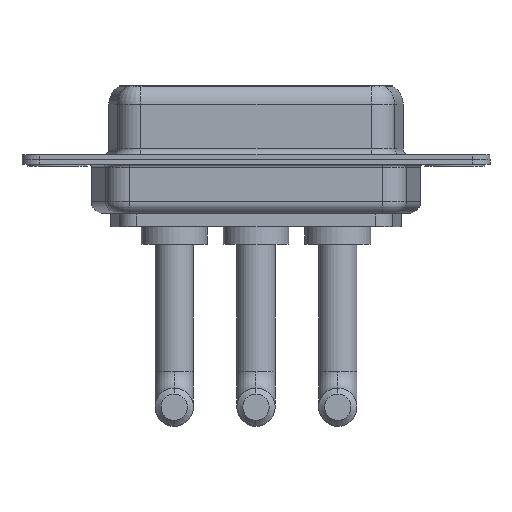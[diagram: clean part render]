
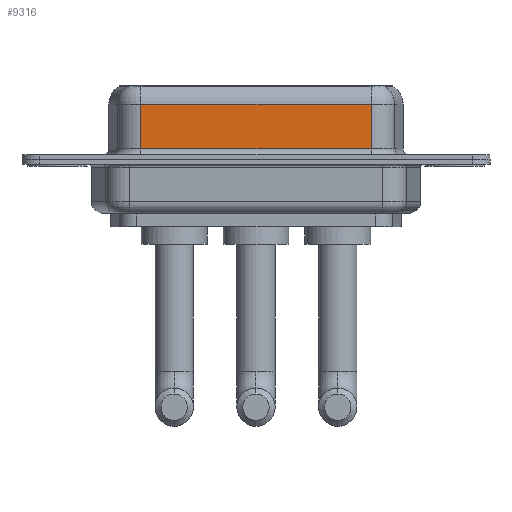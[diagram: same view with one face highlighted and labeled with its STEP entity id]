
A CAD part, front view. The second image highlights one B-rep face of the part: STEP entity #9316.
In plain terms, the highlighted planar face has unit normal (0, -1, 0).
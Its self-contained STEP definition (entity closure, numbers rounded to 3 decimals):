
#898 = PLANE ( 'NONE',  #6904 ) ;
#1173 = CARTESIAN_POINT ( 'NONE',  ( 26.287, -3.95, 0.9 ) ) ;
#2052 = ORIENTED_EDGE ( 'NONE', *, *, #4105, .T. ) ;
#2805 = CARTESIAN_POINT ( 'NONE',  ( 26.287, -3.95, 4.65 ) ) ;
#3080 = EDGE_CURVE ( 'NONE', #8100, #6720, #3349, .T. ) ;
#3349 = LINE ( 'NONE', #9056, #3413 ) ;
#3403 = CARTESIAN_POINT ( 'NONE',  ( 26.287, -3.95, 6.4 ) ) ;
#3413 = VECTOR ( 'NONE', #4997, 1000. ) ;
#3508 = LINE ( 'NONE', #5957, #4964 ) ;
#3719 = LINE ( 'NONE', #9441, #9396 ) ;
#4105 = EDGE_CURVE ( 'NONE', #7250, #8100, #3719, .T. ) ;
#4446 = LINE ( 'NONE', #2805, #8206 ) ;
#4572 = EDGE_CURVE ( 'NONE', #8840, #6720, #3508, .T. ) ;
#4830 = EDGE_LOOP ( 'NONE', ( #8282, #9760, #2052, #8145 ) ) ;
#4964 = VECTOR ( 'NONE', #6760, 1000. ) ;
#4997 = DIRECTION ( 'NONE',  ( 1., 0., 0. ) ) ;
#5092 = DIRECTION ( 'NONE',  ( -1., 0., 0. ) ) ;
#5416 = CARTESIAN_POINT ( 'NONE',  ( 26.287, -3.95, 4.65 ) ) ;
#5427 = CARTESIAN_POINT ( 'NONE',  ( 7.013, -3.95, 4.65 ) ) ;
#5617 = EDGE_CURVE ( 'NONE', #8840, #7250, #4446, .T. ) ;
#5957 = CARTESIAN_POINT ( 'NONE',  ( 26.287, -3.95, 6.4 ) ) ;
#6658 = DIRECTION ( 'NONE',  ( 0., 0., 1. ) ) ;
#6720 = VERTEX_POINT ( 'NONE', #1173 ) ;
#6760 = DIRECTION ( 'NONE',  ( 0., 0., -1. ) ) ;
#6904 = AXIS2_PLACEMENT_3D ( 'NONE', #3403, #8204, #6658 ) ;
#7208 = CARTESIAN_POINT ( 'NONE',  ( 7.013, -3.95, 0.9 ) ) ;
#7250 = VERTEX_POINT ( 'NONE', #5427 ) ;
#8100 = VERTEX_POINT ( 'NONE', #7208 ) ;
#8145 = ORIENTED_EDGE ( 'NONE', *, *, #3080, .T. ) ;
#8204 = DIRECTION ( 'NONE',  ( 0., 1., 0. ) ) ;
#8206 = VECTOR ( 'NONE', #5092, 1000. ) ;
#8282 = ORIENTED_EDGE ( 'NONE', *, *, #4572, .F. ) ;
#8422 = DIRECTION ( 'NONE',  ( 0., 0., -1. ) ) ;
#8840 = VERTEX_POINT ( 'NONE', #5416 ) ;
#9056 = CARTESIAN_POINT ( 'NONE',  ( 26.287, -3.95, 0.9 ) ) ;
#9316 = ADVANCED_FACE ( 'NONE', ( #9819 ), #898, .F. ) ;
#9396 = VECTOR ( 'NONE', #8422, 1000. ) ;
#9441 = CARTESIAN_POINT ( 'NONE',  ( 7.013, -3.95, 6.4 ) ) ;
#9760 = ORIENTED_EDGE ( 'NONE', *, *, #5617, .T. ) ;
#9819 = FACE_OUTER_BOUND ( 'NONE', #4830, .T. ) ;
